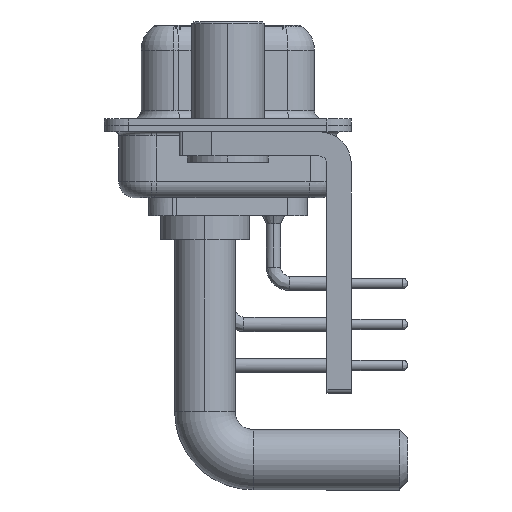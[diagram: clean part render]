
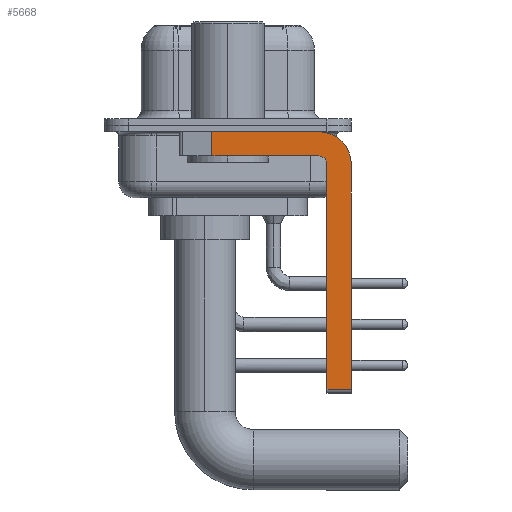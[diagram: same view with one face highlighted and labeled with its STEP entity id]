
A CAD part, left-side view. The second image highlights one B-rep face of the part: STEP entity #5668.
In plain terms, the highlighted planar face has unit normal (-1, 0, 0).
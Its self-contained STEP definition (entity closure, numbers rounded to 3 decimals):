
#21 = DIRECTION ( 'NONE',  ( 0., 0., -1. ) ) ;
#246 = VERTEX_POINT ( 'NONE', #30599 ) ;
#307 = VERTEX_POINT ( 'NONE', #6896 ) ;
#671 = VECTOR ( 'NONE', #21427, 1000. ) ;
#881 = EDGE_CURVE ( 'NONE', #33011, #14374, #1325, .T. ) ;
#1325 = LINE ( 'NONE', #14974, #671 ) ;
#1947 = LINE ( 'NONE', #29252, #5762 ) ;
#2736 = EDGE_LOOP ( 'NONE', ( #10330, #30450, #18178, #35318, #32300, #33892, #25645, #3871 ) ) ;
#3871 = ORIENTED_EDGE ( 'NONE', *, *, #10019, .F. ) ;
#3997 = DIRECTION ( 'NONE',  ( 0., -1., 0. ) ) ;
#4780 = CIRCLE ( 'NONE', #20661, 2. ) ;
#5015 = CARTESIAN_POINT ( 'NONE',  ( -2.9, -5.65, -2.4 ) ) ;
#5476 = CIRCLE ( 'NONE', #9582, 0.5 ) ;
#5577 = LINE ( 'NONE', #16824, #22474 ) ;
#5668 = ADVANCED_FACE ( 'NONE', ( #18649 ), #21627, .F. ) ;
#5712 = EDGE_CURVE ( 'NONE', #36341, #246, #11802, .T. ) ;
#5762 = VECTOR ( 'NONE', #15973, 1000. ) ;
#6215 = CARTESIAN_POINT ( 'NONE',  ( -2.9, -7.65, -16.35 ) ) ;
#6896 = CARTESIAN_POINT ( 'NONE',  ( -2.9, -5.65, -1.9 ) ) ;
#9405 = EDGE_CURVE ( 'NONE', #19340, #10162, #20295, .T. ) ;
#9582 = AXIS2_PLACEMENT_3D ( 'NONE', #28054, #24952, #14048 ) ;
#10019 = EDGE_CURVE ( 'NONE', #33790, #33011, #4780, .T. ) ;
#10162 = VERTEX_POINT ( 'NONE', #35774 ) ;
#10330 = ORIENTED_EDGE ( 'NONE', *, *, #26119, .F. ) ;
#10732 = DIRECTION ( 'NONE',  ( 0., 0., -1. ) ) ;
#11802 = LINE ( 'NONE', #19553, #30444 ) ;
#14048 = DIRECTION ( 'NONE',  ( 0., 0., 1. ) ) ;
#14374 = VERTEX_POINT ( 'NONE', #6215 ) ;
#14974 = CARTESIAN_POINT ( 'NONE',  ( -2.9, -7.65, -2.4 ) ) ;
#15275 = CARTESIAN_POINT ( 'NONE',  ( -2.9, -5.65, -2.4 ) ) ;
#15973 = DIRECTION ( 'NONE',  ( 0., 1., 0. ) ) ;
#16824 = CARTESIAN_POINT ( 'NONE',  ( -2.9, -5.65, -16.35 ) ) ;
#17190 = EDGE_CURVE ( 'NONE', #19340, #14374, #5577, .T. ) ;
#17893 = DIRECTION ( 'NONE',  ( 0., 0., 1. ) ) ;
#18003 = CARTESIAN_POINT ( 'NONE',  ( -2.9, 3., -0.4 ) ) ;
#18178 = ORIENTED_EDGE ( 'NONE', *, *, #24303, .F. ) ;
#18550 = LINE ( 'NONE', #18003, #24102 ) ;
#18649 = FACE_OUTER_BOUND ( 'NONE', #2736, .T. ) ;
#19340 = VERTEX_POINT ( 'NONE', #31355 ) ;
#19553 = CARTESIAN_POINT ( 'NONE',  ( -2.9, 0.978, -1.9 ) ) ;
#20295 = LINE ( 'NONE', #22879, #31837 ) ;
#20661 = AXIS2_PLACEMENT_3D ( 'NONE', #15275, #34849, #20800 ) ;
#20800 = DIRECTION ( 'NONE',  ( 0., 0., -1. ) ) ;
#21074 = CARTESIAN_POINT ( 'NONE',  ( -2.9, -5.65, -0.4 ) ) ;
#21427 = DIRECTION ( 'NONE',  ( 0., 0., -1. ) ) ;
#21627 = PLANE ( 'NONE',  #32784 ) ;
#22018 = DIRECTION ( 'NONE',  ( 0., -1., 0. ) ) ;
#22474 = VECTOR ( 'NONE', #22018, 1000. ) ;
#22879 = CARTESIAN_POINT ( 'NONE',  ( -2.9, -6.15, -16.6 ) ) ;
#24102 = VECTOR ( 'NONE', #3997, 1000. ) ;
#24303 = EDGE_CURVE ( 'NONE', #307, #246, #1947, .T. ) ;
#24766 = DIRECTION ( 'NONE',  ( 1., 0., 0. ) ) ;
#24952 = DIRECTION ( 'NONE',  ( -1., 0., 0. ) ) ;
#25645 = ORIENTED_EDGE ( 'NONE', *, *, #881, .F. ) ;
#26119 = EDGE_CURVE ( 'NONE', #36341, #33790, #18550, .T. ) ;
#28054 = CARTESIAN_POINT ( 'NONE',  ( -2.9, -5.65, -2.4 ) ) ;
#29252 = CARTESIAN_POINT ( 'NONE',  ( -2.9, -5.65, -1.9 ) ) ;
#30318 = CARTESIAN_POINT ( 'NONE',  ( -2.9, 0.978, -0.4 ) ) ;
#30444 = VECTOR ( 'NONE', #21, 1000. ) ;
#30450 = ORIENTED_EDGE ( 'NONE', *, *, #5712, .T. ) ;
#30599 = CARTESIAN_POINT ( 'NONE',  ( -2.9, 0.978, -1.9 ) ) ;
#30924 = CARTESIAN_POINT ( 'NONE',  ( -2.9, -7.65, -2.4 ) ) ;
#31355 = CARTESIAN_POINT ( 'NONE',  ( -2.9, -6.15, -16.35 ) ) ;
#31837 = VECTOR ( 'NONE', #17893, 1000. ) ;
#32300 = ORIENTED_EDGE ( 'NONE', *, *, #9405, .F. ) ;
#32784 = AXIS2_PLACEMENT_3D ( 'NONE', #5015, #24766, #10732 ) ;
#33011 = VERTEX_POINT ( 'NONE', #30924 ) ;
#33790 = VERTEX_POINT ( 'NONE', #21074 ) ;
#33876 = EDGE_CURVE ( 'NONE', #10162, #307, #5476, .T. ) ;
#33892 = ORIENTED_EDGE ( 'NONE', *, *, #17190, .T. ) ;
#34849 = DIRECTION ( 'NONE',  ( 1., 0., 0. ) ) ;
#35318 = ORIENTED_EDGE ( 'NONE', *, *, #33876, .F. ) ;
#35774 = CARTESIAN_POINT ( 'NONE',  ( -2.9, -6.15, -2.4 ) ) ;
#36341 = VERTEX_POINT ( 'NONE', #30318 ) ;
